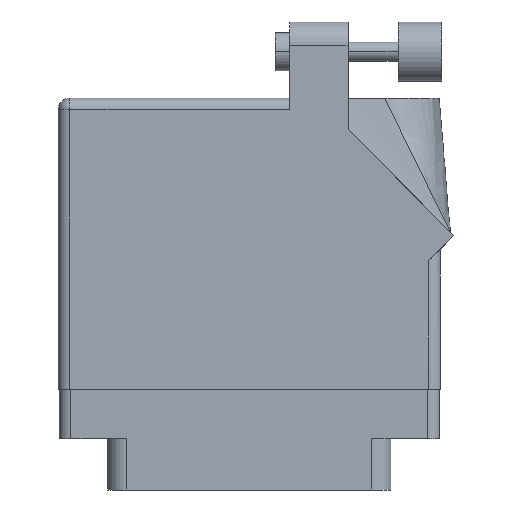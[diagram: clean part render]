
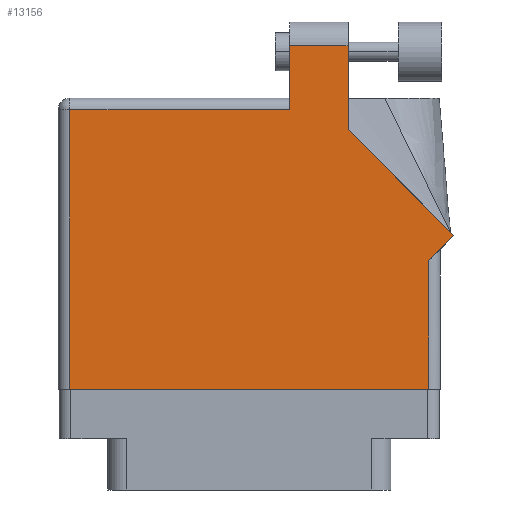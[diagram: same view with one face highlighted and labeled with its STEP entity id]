
A CAD part, front view. The second image highlights one B-rep face of the part: STEP entity #13156.
In plain terms, the highlighted face is planar.
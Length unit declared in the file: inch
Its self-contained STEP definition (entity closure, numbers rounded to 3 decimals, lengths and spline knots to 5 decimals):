
#198 = LINE ( 'NONE', #29091, #29829 ) ;
#802 = VERTEX_POINT ( 'NONE', #19963 ) ;
#2035 = CARTESIAN_POINT ( 'NONE',  ( 1.948, 0., 0. ) ) ;
#2136 = LINE ( 'NONE', #15324, #30060 ) ;
#2184 = DIRECTION ( 'NONE',  ( 0., 0., -1. ) ) ;
#4430 = LINE ( 'NONE', #31372, #10795 ) ;
#4760 = DIRECTION ( 'NONE',  ( 0., -1., 0. ) ) ;
#5679 = CARTESIAN_POINT ( 'NONE',  ( 1.948, 0.675, 0. ) ) ;
#5965 = EDGE_CURVE ( 'NONE', #23755, #22989, #22446, .T. ) ;
#5972 = VERTEX_POINT ( 'NONE', #2035 ) ;
#6882 = DIRECTION ( 'NONE',  ( 0., -1., 0. ) ) ;
#7045 = VERTEX_POINT ( 'NONE', #12579 ) ;
#8298 = VERTEX_POINT ( 'NONE', #9798 ) ;
#9798 = CARTESIAN_POINT ( 'NONE',  ( 1.217, 1.805, 0. ) ) ;
#9927 = ORIENTED_EDGE ( 'NONE', *, *, #24222, .T. ) ;
#10101 = DIRECTION ( 'NONE',  ( 0., 1., 0. ) ) ;
#10783 = LINE ( 'NONE', #10966, #33633 ) ;
#10795 = VECTOR ( 'NONE', #4760, 39.37008 ) ;
#10966 = CARTESIAN_POINT ( 'NONE',  ( 2.01, 0.737, 0. ) ) ;
#11656 = LINE ( 'NONE', #30079, #22212 ) ;
#12414 = EDGE_CURVE ( 'NONE', #28587, #7045, #29072, .T. ) ;
#12579 = CARTESIAN_POINT ( 'NONE',  ( 0.062, 0., 0. ) ) ;
#12738 = LINE ( 'NONE', #21648, #14908 ) ;
#13156 = ADVANCED_FACE ( 'NONE', ( #22681 ), #31979, .F. ) ;
#13212 = ORIENTED_EDGE ( 'NONE', *, *, #24018, .T. ) ;
#13448 = AXIS2_PLACEMENT_3D ( 'NONE', #31864, #2184, #21246 ) ;
#13705 = DIRECTION ( 'NONE',  ( 0.707, 0.707, 0. ) ) ;
#13935 = DIRECTION ( 'NONE',  ( 1., 0., 0. ) ) ;
#14481 = VERTEX_POINT ( 'NONE', #5679 ) ;
#14908 = VECTOR ( 'NONE', #24919, 39.37008 ) ;
#14921 = ORIENTED_EDGE ( 'NONE', *, *, #21399, .T. ) ;
#15324 = CARTESIAN_POINT ( 'NONE',  ( 1.217, 1.805, 0. ) ) ;
#16965 = EDGE_CURVE ( 'NONE', #7045, #5972, #11656, .T. ) ;
#17142 = EDGE_CURVE ( 'NONE', #8298, #19908, #4430, .T. ) ;
#19602 = VECTOR ( 'NONE', #29737, 39.37008 ) ;
#19908 = VERTEX_POINT ( 'NONE', #33057 ) ;
#19963 = CARTESIAN_POINT ( 'NONE',  ( 1.524, 1.805, 0. ) ) ;
#20127 = EDGE_LOOP ( 'NONE', ( #27576, #13212, #29760, #9927, #21507, #25669, #31183, #14921, #26960 ) ) ;
#21246 = DIRECTION ( 'NONE',  ( -1., 0., 0. ) ) ;
#21399 = EDGE_CURVE ( 'NONE', #14481, #23755, #10783, .T. ) ;
#21501 = CARTESIAN_POINT ( 'NONE',  ( 1.948, 0.737, 0. ) ) ;
#21507 = ORIENTED_EDGE ( 'NONE', *, *, #12414, .T. ) ;
#21648 = CARTESIAN_POINT ( 'NONE',  ( 0., 1.468, 0. ) ) ;
#22212 = VECTOR ( 'NONE', #13935, 39.37008 ) ;
#22446 = LINE ( 'NONE', #29216, #30890 ) ;
#22681 = FACE_OUTER_BOUND ( 'NONE', #20127, .T. ) ;
#22987 = EDGE_CURVE ( 'NONE', #5972, #14481, #26799, .T. ) ;
#22989 = VERTEX_POINT ( 'NONE', #29627 ) ;
#23055 = CARTESIAN_POINT ( 'NONE',  ( 0.062, 0., 0. ) ) ;
#23755 = VERTEX_POINT ( 'NONE', #32995 ) ;
#24018 = EDGE_CURVE ( 'NONE', #802, #8298, #2136, .T. ) ;
#24222 = EDGE_CURVE ( 'NONE', #19908, #28587, #12738, .T. ) ;
#24919 = DIRECTION ( 'NONE',  ( -1., 0., 0. ) ) ;
#25669 = ORIENTED_EDGE ( 'NONE', *, *, #16965, .T. ) ;
#26537 = CARTESIAN_POINT ( 'NONE',  ( 0.062, 1.468, 0. ) ) ;
#26799 = LINE ( 'NONE', #21501, #19602 ) ;
#26960 = ORIENTED_EDGE ( 'NONE', *, *, #5965, .T. ) ;
#27576 = ORIENTED_EDGE ( 'NONE', *, *, #31488, .T. ) ;
#28587 = VERTEX_POINT ( 'NONE', #26537 ) ;
#29072 = LINE ( 'NONE', #23055, #33740 ) ;
#29091 = CARTESIAN_POINT ( 'NONE',  ( 1.524, 1.36442, 0. ) ) ;
#29216 = CARTESIAN_POINT ( 'NONE',  ( 2.08071, 0.80771, 0. ) ) ;
#29627 = CARTESIAN_POINT ( 'NONE',  ( 1.524, 1.36442, 0. ) ) ;
#29737 = DIRECTION ( 'NONE',  ( 0., 1., 0. ) ) ;
#29760 = ORIENTED_EDGE ( 'NONE', *, *, #17142, .T. ) ;
#29829 = VECTOR ( 'NONE', #10101, 39.37008 ) ;
#30060 = VECTOR ( 'NONE', #31566, 39.37008 ) ;
#30079 = CARTESIAN_POINT ( 'NONE',  ( 0., 0., 0. ) ) ;
#30890 = VECTOR ( 'NONE', #34438, 39.37008 ) ;
#31183 = ORIENTED_EDGE ( 'NONE', *, *, #22987, .T. ) ;
#31372 = CARTESIAN_POINT ( 'NONE',  ( 1.217, 1.53, 0. ) ) ;
#31488 = EDGE_CURVE ( 'NONE', #22989, #802, #198, .T. ) ;
#31566 = DIRECTION ( 'NONE',  ( -1., 0., 0. ) ) ;
#31864 = CARTESIAN_POINT ( 'NONE',  ( 0., 1.53, 0. ) ) ;
#31979 = PLANE ( 'NONE',  #13448 ) ;
#32995 = CARTESIAN_POINT ( 'NONE',  ( 2.08071, 0.80771, 0. ) ) ;
#33057 = CARTESIAN_POINT ( 'NONE',  ( 1.217, 1.468, 0. ) ) ;
#33633 = VECTOR ( 'NONE', #13705, 39.37008 ) ;
#33740 = VECTOR ( 'NONE', #6882, 39.37008 ) ;
#34438 = DIRECTION ( 'NONE',  ( -0.707, 0.707, 0. ) ) ;
